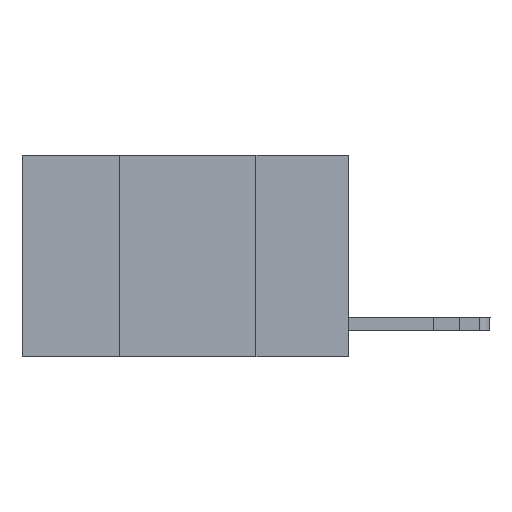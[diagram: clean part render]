
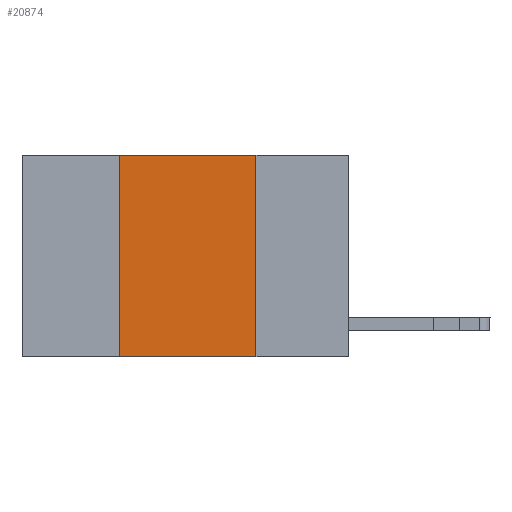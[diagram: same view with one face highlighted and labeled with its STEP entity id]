
A CAD part, left-side view. The second image highlights one B-rep face of the part: STEP entity #20874.
In plain terms, the highlighted planar face has unit normal (-1, 0, 0).
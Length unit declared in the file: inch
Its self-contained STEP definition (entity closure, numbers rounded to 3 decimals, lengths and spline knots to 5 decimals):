
#128 = VERTEX_POINT ( 'NONE', #9949 ) ;
#661 = DIRECTION ( 'NONE',  ( 0., -1., 0. ) ) ;
#1243 = DIRECTION ( 'NONE',  ( 0., 0., -1. ) ) ;
#1873 = DIRECTION ( 'NONE',  ( 0., 0., 1. ) ) ;
#2162 = PLANE ( 'NONE',  #16387 ) ;
#2612 = CARTESIAN_POINT ( 'NONE',  ( 0., 0.17, -0.37 ) ) ;
#3597 = VECTOR ( 'NONE', #1873, 39.37008 ) ;
#3765 = EDGE_CURVE ( 'NONE', #13908, #128, #12612, .T. ) ;
#5920 = EDGE_CURVE ( 'NONE', #128, #22956, #10332, .T. ) ;
#7375 = VECTOR ( 'NONE', #661, 39.37008 ) ;
#8191 = DIRECTION ( 'NONE',  ( 1., 0., 0. ) ) ;
#9418 = ORIENTED_EDGE ( 'NONE', *, *, #25117, .T. ) ;
#9949 = CARTESIAN_POINT ( 'NONE',  ( 0., 0.17, 0. ) ) ;
#10332 = LINE ( 'NONE', #22624, #14849 ) ;
#11264 = EDGE_LOOP ( 'NONE', ( #21505, #13836, #20160, #9418 ) ) ;
#12546 = LINE ( 'NONE', #16278, #7375 ) ;
#12612 = LINE ( 'NONE', #22954, #18277 ) ;
#12707 = EDGE_CURVE ( 'NONE', #21308, #13908, #23549, .T. ) ;
#13836 = ORIENTED_EDGE ( 'NONE', *, *, #3765, .F. ) ;
#13908 = VERTEX_POINT ( 'NONE', #19794 ) ;
#13951 = CARTESIAN_POINT ( 'NONE',  ( 0., 0.6, 0. ) ) ;
#14849 = VECTOR ( 'NONE', #1243, 39.37008 ) ;
#15675 = CARTESIAN_POINT ( 'NONE',  ( 0., 0.42, 0. ) ) ;
#16278 = CARTESIAN_POINT ( 'NONE',  ( 0., 0.6, -0.37 ) ) ;
#16387 = AXIS2_PLACEMENT_3D ( 'NONE', #13951, #8191, #21582 ) ;
#18277 = VECTOR ( 'NONE', #24857, 39.37008 ) ;
#19794 = CARTESIAN_POINT ( 'NONE',  ( 0., 0.42, 0. ) ) ;
#20160 = ORIENTED_EDGE ( 'NONE', *, *, #12707, .F. ) ;
#20874 = ADVANCED_FACE ( 'NONE', ( #22275 ), #2162, .F. ) ;
#21308 = VERTEX_POINT ( 'NONE', #25169 ) ;
#21505 = ORIENTED_EDGE ( 'NONE', *, *, #5920, .F. ) ;
#21582 = DIRECTION ( 'NONE',  ( 0., 0., -1. ) ) ;
#22275 = FACE_OUTER_BOUND ( 'NONE', #11264, .T. ) ;
#22624 = CARTESIAN_POINT ( 'NONE',  ( 0., 0.17, 0. ) ) ;
#22954 = CARTESIAN_POINT ( 'NONE',  ( 0., 0.6, 0. ) ) ;
#22956 = VERTEX_POINT ( 'NONE', #2612 ) ;
#23549 = LINE ( 'NONE', #15675, #3597 ) ;
#24857 = DIRECTION ( 'NONE',  ( 0., -1., 0. ) ) ;
#25117 = EDGE_CURVE ( 'NONE', #21308, #22956, #12546, .T. ) ;
#25169 = CARTESIAN_POINT ( 'NONE',  ( 0., 0.42, -0.37 ) ) ;
